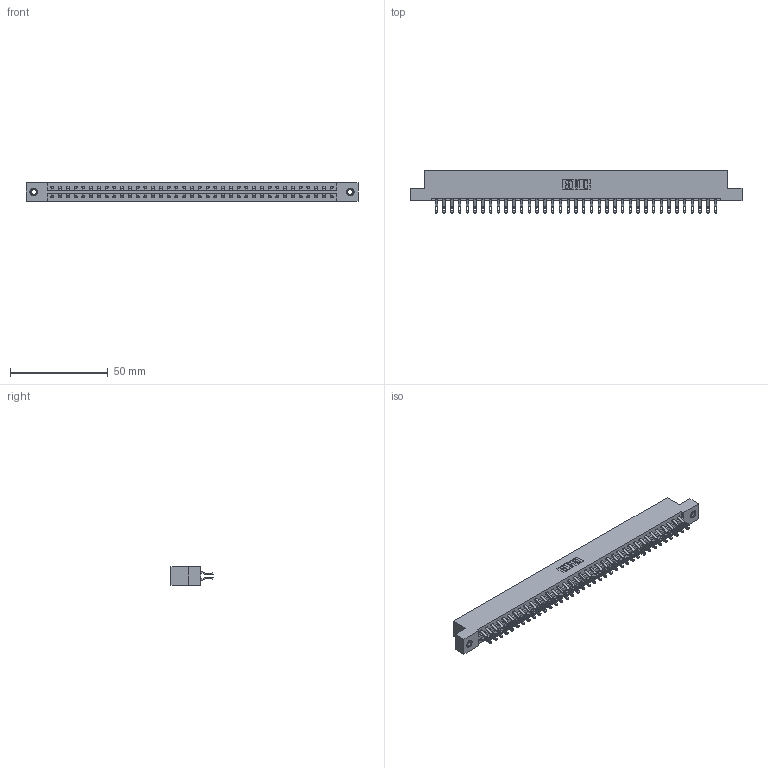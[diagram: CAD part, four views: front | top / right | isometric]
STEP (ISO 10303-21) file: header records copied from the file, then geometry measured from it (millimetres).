
FILE_DESCRIPTION (( 'STEP AP203' ), '1' );
FILE_NAME ('387-074-555-207.STEP', '2019-10-22T02:09:38', ( '' ), ( '' ), 'SwSTEP 2.0', 'SolidWorks 2016', '' );
FILE_SCHEMA (( 'CONFIG_CONTROL_DESIGN' ));
Length unit declared in the file: inch
Products named in the file (4): 387-074-555-207; 345-250-001_345-250-005-103; 345-292-001_555 Tail; 337 Part_Flush Mounting Lugs - 0.156 Dia-TI
Assembly tree (77 placements, depth 2):
  387-074-555-207
    337 Part_Flush Mounting Lugs - 0.156 Dia-TI
    345-292-001_555 Tail  x74
    345-250-001_345-250-005-103  x2
Bounding box: 169.62 x 21.47 x 9.4 mm (x, y, z)
Volume: 18010.6 mm3; surface area: 21157.3 mm2
Topology: 77 solids, 77 shells, 4614 faces, 14433 edges, 9614 vertices
Faces by surface type: plane 2766, cylinder 1832, cone 12, torus 4
Entity records: 30846 total; most frequent: CARTESIAN_POINT 5215, ORIENTED_EDGE 5114, DIRECTION 4447, EDGE_CURVE 2557, LINE 2389, VECTOR 2389, VERTEX_POINT 1700, AXIS2_PLACEMENT_3D 1029
